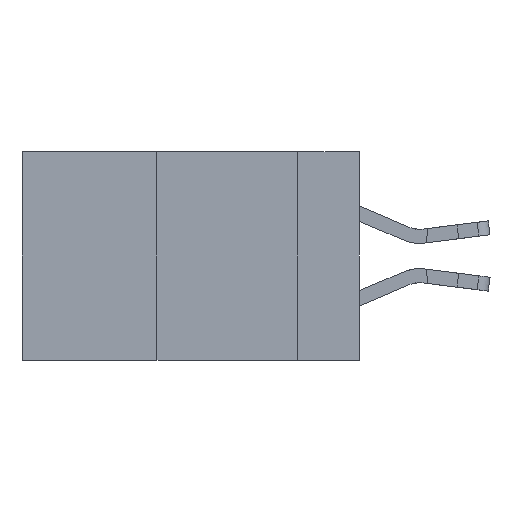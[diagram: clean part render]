
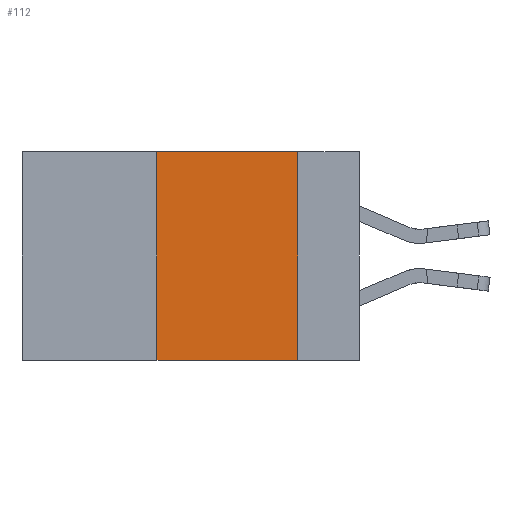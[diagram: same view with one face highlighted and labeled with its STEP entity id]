
A CAD part, left-side view. The second image highlights one B-rep face of the part: STEP entity #112.
In plain terms, the highlighted planar face has unit normal (-1, 0, 0).
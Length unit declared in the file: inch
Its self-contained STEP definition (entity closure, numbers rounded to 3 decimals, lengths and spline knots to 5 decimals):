
#21 = ORIENTED_EDGE ( 'NONE', *, *, #15581, .F. ) ;
#112 = ADVANCED_FACE ( 'NONE', ( #7499 ), #5629, .F. ) ;
#1425 = ORIENTED_EDGE ( 'NONE', *, *, #7065, .F. ) ;
#2531 = DIRECTION ( 'NONE',  ( 1., 0., 0. ) ) ;
#3341 = VERTEX_POINT ( 'NONE', #24834 ) ;
#5042 = CARTESIAN_POINT ( 'NONE',  ( 0., 0.11, -0.37 ) ) ;
#5629 = PLANE ( 'NONE',  #7982 ) ;
#5809 = VERTEX_POINT ( 'NONE', #5042 ) ;
#6074 = VERTEX_POINT ( 'NONE', #22900 ) ;
#6385 = LINE ( 'NONE', #22285, #26775 ) ;
#6912 = EDGE_CURVE ( 'NONE', #6074, #19148, #12345, .T. ) ;
#7065 = EDGE_CURVE ( 'NONE', #19148, #3341, #10286, .T. ) ;
#7177 = DIRECTION ( 'NONE',  ( 0., 0., -1. ) ) ;
#7499 = FACE_OUTER_BOUND ( 'NONE', #25299, .T. ) ;
#7982 = AXIS2_PLACEMENT_3D ( 'NONE', #10631, #2531, #9066 ) ;
#8585 = ORIENTED_EDGE ( 'NONE', *, *, #21620, .T. ) ;
#9065 = CARTESIAN_POINT ( 'NONE',  ( 0., 0.6, 0. ) ) ;
#9066 = DIRECTION ( 'NONE',  ( 0., 0., -1. ) ) ;
#10286 = LINE ( 'NONE', #9065, #24994 ) ;
#10631 = CARTESIAN_POINT ( 'NONE',  ( 0., 0.6, 0. ) ) ;
#12345 = LINE ( 'NONE', #21215, #22751 ) ;
#13024 = ORIENTED_EDGE ( 'NONE', *, *, #6912, .F. ) ;
#15581 = EDGE_CURVE ( 'NONE', #3341, #5809, #16726, .T. ) ;
#16072 = VECTOR ( 'NONE', #7177, 39.37008 ) ;
#16726 = LINE ( 'NONE', #17832, #16072 ) ;
#16956 = CARTESIAN_POINT ( 'NONE',  ( 0., 0.36, 0. ) ) ;
#17832 = CARTESIAN_POINT ( 'NONE',  ( 0., 0.11, 0. ) ) ;
#19148 = VERTEX_POINT ( 'NONE', #16956 ) ;
#20302 = DIRECTION ( 'NONE',  ( 0., -1., 0. ) ) ;
#21215 = CARTESIAN_POINT ( 'NONE',  ( 0., 0.36, 0. ) ) ;
#21620 = EDGE_CURVE ( 'NONE', #6074, #5809, #6385, .T. ) ;
#22285 = CARTESIAN_POINT ( 'NONE',  ( 0., 0.6, -0.37 ) ) ;
#22751 = VECTOR ( 'NONE', #25365, 39.37008 ) ;
#22900 = CARTESIAN_POINT ( 'NONE',  ( 0., 0.36, -0.37 ) ) ;
#24834 = CARTESIAN_POINT ( 'NONE',  ( 0., 0.11, 0. ) ) ;
#24994 = VECTOR ( 'NONE', #25827, 39.37008 ) ;
#25299 = EDGE_LOOP ( 'NONE', ( #21, #1425, #13024, #8585 ) ) ;
#25365 = DIRECTION ( 'NONE',  ( 0., 0., 1. ) ) ;
#25827 = DIRECTION ( 'NONE',  ( 0., -1., 0. ) ) ;
#26775 = VECTOR ( 'NONE', #20302, 39.37008 ) ;
